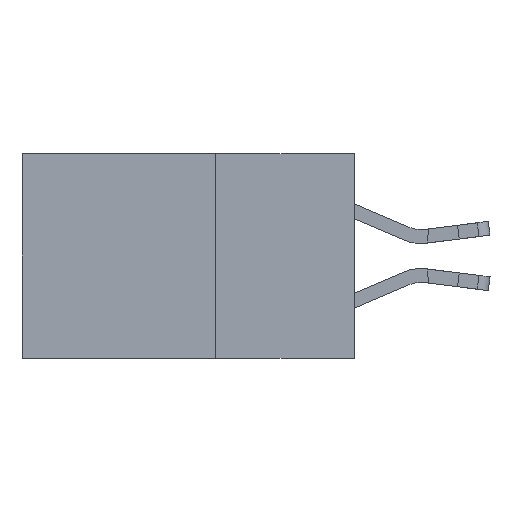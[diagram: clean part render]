
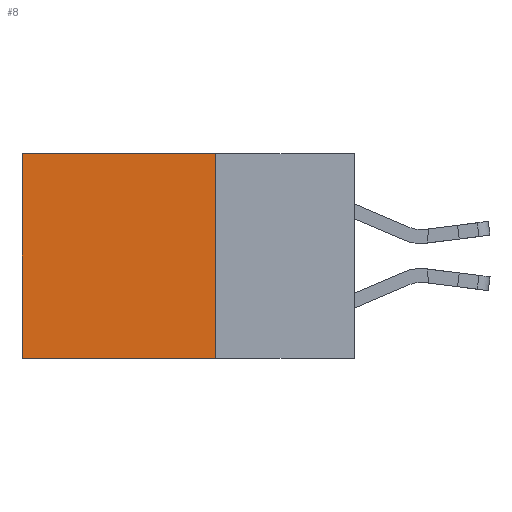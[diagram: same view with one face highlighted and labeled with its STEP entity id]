
A CAD part, left-side view. The second image highlights one B-rep face of the part: STEP entity #8.
In plain terms, the highlighted planar face has unit normal (-1, 0, 0).
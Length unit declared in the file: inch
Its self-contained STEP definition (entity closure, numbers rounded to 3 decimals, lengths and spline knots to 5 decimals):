
#8 = ADVANCED_FACE ( 'NONE', ( #13742 ), #1446, .F. ) ;
#524 = VERTEX_POINT ( 'NONE', #16446 ) ;
#1125 = VECTOR ( 'NONE', #7835, 39.37008 ) ;
#1446 = PLANE ( 'NONE',  #14949 ) ;
#3599 = VERTEX_POINT ( 'NONE', #14531 ) ;
#3608 = LINE ( 'NONE', #15817, #13640 ) ;
#3710 = ORIENTED_EDGE ( 'NONE', *, *, #13766, .F. ) ;
#3765 = DIRECTION ( 'NONE',  ( 0., 0., -1. ) ) ;
#4038 = DIRECTION ( 'NONE',  ( 0., 1., 0. ) ) ;
#4261 = DIRECTION ( 'NONE',  ( 0., 0., -1. ) ) ;
#4401 = CARTESIAN_POINT ( 'NONE',  ( 0.298, 0.6, -0.37 ) ) ;
#4895 = CARTESIAN_POINT ( 'NONE',  ( 0.298, 0.6, 0. ) ) ;
#5032 = LINE ( 'NONE', #4895, #9058 ) ;
#7168 = LINE ( 'NONE', #11680, #1125 ) ;
#7580 = EDGE_LOOP ( 'NONE', ( #8704, #3710, #14936, #10098 ) ) ;
#7835 = DIRECTION ( 'NONE',  ( 0., 1., 0. ) ) ;
#8301 = VERTEX_POINT ( 'NONE', #4401 ) ;
#8704 = ORIENTED_EDGE ( 'NONE', *, *, #14347, .T. ) ;
#9058 = VECTOR ( 'NONE', #3765, 39.37008 ) ;
#9416 = EDGE_CURVE ( 'NONE', #13847, #3599, #7168, .T. ) ;
#10098 = ORIENTED_EDGE ( 'NONE', *, *, #9416, .T. ) ;
#10452 = DIRECTION ( 'NONE',  ( 1., 0., 0. ) ) ;
#10741 = LINE ( 'NONE', #13152, #15125 ) ;
#11034 = EDGE_CURVE ( 'NONE', #13847, #524, #3608, .T. ) ;
#11680 = CARTESIAN_POINT ( 'NONE',  ( 0.298, 0.25, 0. ) ) ;
#13152 = CARTESIAN_POINT ( 'NONE',  ( 0.298, 0.25, -0.37 ) ) ;
#13206 = CARTESIAN_POINT ( 'NONE',  ( 0.298, 0.25, 0. ) ) ;
#13264 = CARTESIAN_POINT ( 'NONE',  ( 0.298, 0.25, 0. ) ) ;
#13640 = VECTOR ( 'NONE', #14839, 39.37008 ) ;
#13742 = FACE_OUTER_BOUND ( 'NONE', #7580, .T. ) ;
#13766 = EDGE_CURVE ( 'NONE', #524, #8301, #10741, .T. ) ;
#13847 = VERTEX_POINT ( 'NONE', #13264 ) ;
#14347 = EDGE_CURVE ( 'NONE', #3599, #8301, #5032, .T. ) ;
#14531 = CARTESIAN_POINT ( 'NONE',  ( 0.298, 0.6, 0. ) ) ;
#14839 = DIRECTION ( 'NONE',  ( 0., 0., -1. ) ) ;
#14936 = ORIENTED_EDGE ( 'NONE', *, *, #11034, .F. ) ;
#14949 = AXIS2_PLACEMENT_3D ( 'NONE', #13206, #10452, #4261 ) ;
#15125 = VECTOR ( 'NONE', #4038, 39.37008 ) ;
#15817 = CARTESIAN_POINT ( 'NONE',  ( 0.298, 0.25, 0. ) ) ;
#16446 = CARTESIAN_POINT ( 'NONE',  ( 0.298, 0.25, -0.37 ) ) ;
